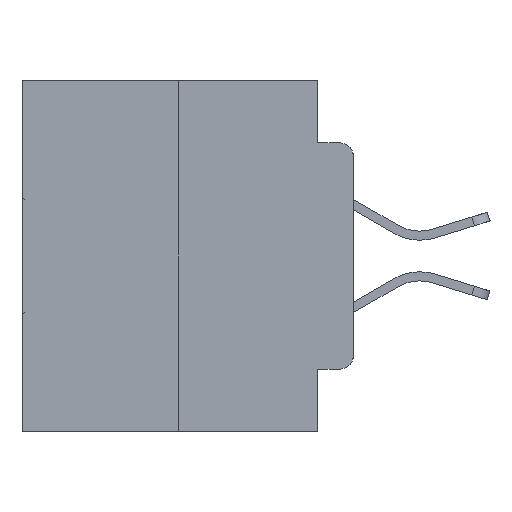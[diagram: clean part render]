
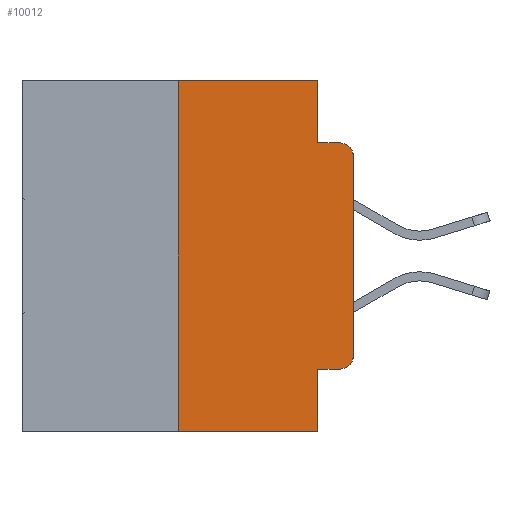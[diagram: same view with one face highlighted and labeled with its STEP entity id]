
A CAD part, left-side view. The second image highlights one B-rep face of the part: STEP entity #10012.
In plain terms, the highlighted planar face has unit normal (-1, 0, 0).
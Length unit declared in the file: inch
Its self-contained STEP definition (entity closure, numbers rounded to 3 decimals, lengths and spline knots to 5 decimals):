
#46 = FACE_OUTER_BOUND ( 'NONE', #27072, .T. ) ;
#860 = CARTESIAN_POINT ( 'NONE',  ( 0., 0.25, 0. ) ) ;
#1146 = DIRECTION ( 'NONE',  ( 0., -1., 0. ) ) ;
#1223 = VECTOR ( 'NONE', #8774, 39.37008 ) ;
#1564 = LINE ( 'NONE', #860, #13729 ) ;
#2140 = CARTESIAN_POINT ( 'NONE',  ( 0., 0., -0.3915 ) ) ;
#2235 = EDGE_CURVE ( 'NONE', #3570, #10889, #16549, .T. ) ;
#2357 = CARTESIAN_POINT ( 'NONE',  ( 0., 0.02, -0.3915 ) ) ;
#2498 = LINE ( 'NONE', #26448, #3247 ) ;
#2860 = VECTOR ( 'NONE', #1146, 39.37008 ) ;
#3087 = LINE ( 'NONE', #24383, #25448 ) ;
#3210 = DIRECTION ( 'NONE',  ( 0., 0., 1. ) ) ;
#3247 = VECTOR ( 'NONE', #11030, 39.37008 ) ;
#3448 = DIRECTION ( 'NONE',  ( -1., 0., 0. ) ) ;
#3569 = AXIS2_PLACEMENT_3D ( 'NONE', #17040, #3448, #19212 ) ;
#3570 = VERTEX_POINT ( 'NONE', #26144 ) ;
#3759 = CARTESIAN_POINT ( 'NONE',  ( 0., 0.473, 0. ) ) ;
#3906 = CARTESIAN_POINT ( 'NONE',  ( 0., 0.02, -0.0885 ) ) ;
#4093 = ORIENTED_EDGE ( 'NONE', *, *, #15174, .T. ) ;
#4231 = CARTESIAN_POINT ( 'NONE',  ( 0., 0.25, -0.5 ) ) ;
#4633 = VERTEX_POINT ( 'NONE', #9866 ) ;
#4709 = DIRECTION ( 'NONE',  ( 0., 0., -1. ) ) ;
#4980 = CIRCLE ( 'NONE', #3569, 0.02 ) ;
#7263 = EDGE_CURVE ( 'NONE', #4633, #10889, #4980, .T. ) ;
#7387 = EDGE_CURVE ( 'NONE', #27774, #13504, #7464, .T. ) ;
#7464 = LINE ( 'NONE', #3759, #19401 ) ;
#7662 = ORIENTED_EDGE ( 'NONE', *, *, #2235, .F. ) ;
#7693 = ORIENTED_EDGE ( 'NONE', *, *, #7387, .F. ) ;
#7912 = CARTESIAN_POINT ( 'NONE',  ( 0., 0.02, -0.4115 ) ) ;
#7999 = CARTESIAN_POINT ( 'NONE',  ( 0., 0.473, -0.5 ) ) ;
#8038 = ORIENTED_EDGE ( 'NONE', *, *, #12144, .F. ) ;
#8774 = DIRECTION ( 'NONE',  ( 0., 0., 1. ) ) ;
#8970 = LINE ( 'NONE', #7999, #2860 ) ;
#9143 = ORIENTED_EDGE ( 'NONE', *, *, #22494, .F. ) ;
#9174 = VECTOR ( 'NONE', #9798, 39.37008 ) ;
#9798 = DIRECTION ( 'NONE',  ( 0., 0., -1. ) ) ;
#9866 = CARTESIAN_POINT ( 'NONE',  ( 0., 0., -0.1085 ) ) ;
#10012 = ADVANCED_FACE ( 'NONE', ( #46 ), #16555, .F. ) ;
#10889 = VERTEX_POINT ( 'NONE', #3906 ) ;
#11030 = DIRECTION ( 'NONE',  ( 0., 0., -1. ) ) ;
#11965 = ORIENTED_EDGE ( 'NONE', *, *, #18409, .T. ) ;
#12106 = DIRECTION ( 'NONE',  ( 0., 0., -1. ) ) ;
#12144 = EDGE_CURVE ( 'NONE', #13504, #3570, #2498, .T. ) ;
#13221 = CARTESIAN_POINT ( 'NONE',  ( 0., 0.051, -0.4115 ) ) ;
#13447 = DIRECTION ( 'NONE',  ( 0., -1., 0. ) ) ;
#13504 = VERTEX_POINT ( 'NONE', #13619 ) ;
#13619 = CARTESIAN_POINT ( 'NONE',  ( 0., 0.051, 0. ) ) ;
#13729 = VECTOR ( 'NONE', #3210, 39.37008 ) ;
#13843 = AXIS2_PLACEMENT_3D ( 'NONE', #2357, #18211, #4709 ) ;
#14083 = ORIENTED_EDGE ( 'NONE', *, *, #14876, .F. ) ;
#14876 = EDGE_CURVE ( 'NONE', #17352, #15944, #21012, .T. ) ;
#15174 = EDGE_CURVE ( 'NONE', #18678, #4633, #17256, .T. ) ;
#15227 = AXIS2_PLACEMENT_3D ( 'NONE', #20918, #25286, #12106 ) ;
#15944 = VERTEX_POINT ( 'NONE', #26640 ) ;
#16331 = VERTEX_POINT ( 'NONE', #7912 ) ;
#16549 = LINE ( 'NONE', #18608, #21640 ) ;
#16555 = PLANE ( 'NONE',  #15227 ) ;
#16617 = CARTESIAN_POINT ( 'NONE',  ( 0., 0.051, 0. ) ) ;
#16694 = EDGE_CURVE ( 'NONE', #16331, #18678, #27406, .T. ) ;
#17040 = CARTESIAN_POINT ( 'NONE',  ( 0., 0.02, -0.1085 ) ) ;
#17256 = LINE ( 'NONE', #22085, #1223 ) ;
#17352 = VERTEX_POINT ( 'NONE', #13221 ) ;
#18175 = DIRECTION ( 'NONE',  ( 0., -1., 0. ) ) ;
#18211 = DIRECTION ( 'NONE',  ( -1., 0., 0. ) ) ;
#18409 = EDGE_CURVE ( 'NONE', #24840, #15944, #8970, .T. ) ;
#18608 = CARTESIAN_POINT ( 'NONE',  ( 0., 0.051, -0.0885 ) ) ;
#18678 = VERTEX_POINT ( 'NONE', #2140 ) ;
#19212 = DIRECTION ( 'NONE',  ( 0., 0., -1. ) ) ;
#19401 = VECTOR ( 'NONE', #26065, 39.37008 ) ;
#19953 = ORIENTED_EDGE ( 'NONE', *, *, #27144, .T. ) ;
#20918 = CARTESIAN_POINT ( 'NONE',  ( 0., 0.473, 0. ) ) ;
#21012 = LINE ( 'NONE', #16617, #9174 ) ;
#21329 = ORIENTED_EDGE ( 'NONE', *, *, #16694, .T. ) ;
#21640 = VECTOR ( 'NONE', #18175, 39.37008 ) ;
#21949 = ORIENTED_EDGE ( 'NONE', *, *, #7263, .T. ) ;
#22085 = CARTESIAN_POINT ( 'NONE',  ( 0., 0., 0. ) ) ;
#22494 = EDGE_CURVE ( 'NONE', #24840, #27774, #1564, .T. ) ;
#24383 = CARTESIAN_POINT ( 'NONE',  ( 0., 0.051, -0.4115 ) ) ;
#24743 = CARTESIAN_POINT ( 'NONE',  ( 0., 0.25, 0. ) ) ;
#24840 = VERTEX_POINT ( 'NONE', #4231 ) ;
#25286 = DIRECTION ( 'NONE',  ( 1., 0., 0. ) ) ;
#25448 = VECTOR ( 'NONE', #13447, 39.37008 ) ;
#26065 = DIRECTION ( 'NONE',  ( 0., -1., 0. ) ) ;
#26144 = CARTESIAN_POINT ( 'NONE',  ( 0., 0.051, -0.0885 ) ) ;
#26448 = CARTESIAN_POINT ( 'NONE',  ( 0., 0.051, 0. ) ) ;
#26640 = CARTESIAN_POINT ( 'NONE',  ( 0., 0.051, -0.5 ) ) ;
#27072 = EDGE_LOOP ( 'NONE', ( #4093, #21949, #7662, #8038, #7693, #9143, #11965, #14083, #19953, #21329 ) ) ;
#27144 = EDGE_CURVE ( 'NONE', #17352, #16331, #3087, .T. ) ;
#27406 = CIRCLE ( 'NONE', #13843, 0.02 ) ;
#27774 = VERTEX_POINT ( 'NONE', #24743 ) ;
